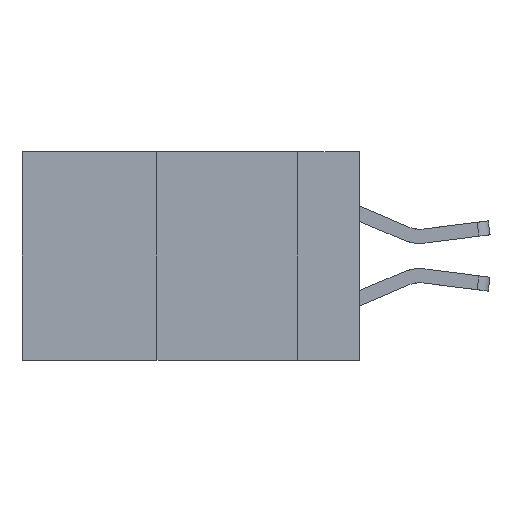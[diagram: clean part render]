
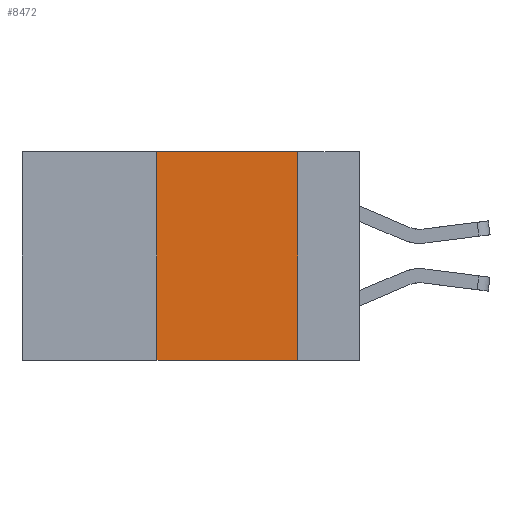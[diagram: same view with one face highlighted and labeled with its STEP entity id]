
A CAD part, left-side view. The second image highlights one B-rep face of the part: STEP entity #8472.
In plain terms, the highlighted planar face has unit normal (-1, 0, 0).
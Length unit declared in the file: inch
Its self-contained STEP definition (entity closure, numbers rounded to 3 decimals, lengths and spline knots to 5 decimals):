
#332 = DIRECTION ( 'NONE',  ( 0., 0., 1. ) ) ;
#389 = DIRECTION ( 'NONE',  ( 0., 0., -1. ) ) ;
#1314 = EDGE_CURVE ( 'NONE', #3086, #7389, #4109, .T. ) ;
#1428 = ORIENTED_EDGE ( 'NONE', *, *, #9769, .F. ) ;
#1453 = VERTEX_POINT ( 'NONE', #2258 ) ;
#2258 = CARTESIAN_POINT ( 'NONE',  ( 0., 0.36, 0. ) ) ;
#2294 = LINE ( 'NONE', #9237, #9039 ) ;
#3086 = VERTEX_POINT ( 'NONE', #4853 ) ;
#3534 = EDGE_CURVE ( 'NONE', #3086, #1453, #8638, .T. ) ;
#3850 = ORIENTED_EDGE ( 'NONE', *, *, #1314, .T. ) ;
#3975 = DIRECTION ( 'NONE',  ( 0., -1., 0. ) ) ;
#4109 = LINE ( 'NONE', #9462, #5399 ) ;
#4118 = CARTESIAN_POINT ( 'NONE',  ( 0., 0.6, 0. ) ) ;
#4625 = DIRECTION ( 'NONE',  ( 0., 0., -1. ) ) ;
#4808 = CARTESIAN_POINT ( 'NONE',  ( 0., 0.11, -0.37 ) ) ;
#4853 = CARTESIAN_POINT ( 'NONE',  ( 0., 0.36, -0.37 ) ) ;
#4981 = LINE ( 'NONE', #5842, #8433 ) ;
#5399 = VECTOR ( 'NONE', #6715, 39.37008 ) ;
#5842 = CARTESIAN_POINT ( 'NONE',  ( 0., 0.6, 0. ) ) ;
#6715 = DIRECTION ( 'NONE',  ( 0., -1., 0. ) ) ;
#6769 = ORIENTED_EDGE ( 'NONE', *, *, #9704, .F. ) ;
#6993 = ORIENTED_EDGE ( 'NONE', *, *, #3534, .F. ) ;
#7389 = VERTEX_POINT ( 'NONE', #4808 ) ;
#8433 = VECTOR ( 'NONE', #3975, 39.37008 ) ;
#8457 = VERTEX_POINT ( 'NONE', #10079 ) ;
#8472 = ADVANCED_FACE ( 'NONE', ( #11332 ), #8593, .F. ) ;
#8576 = CARTESIAN_POINT ( 'NONE',  ( 0., 0.36, 0. ) ) ;
#8593 = PLANE ( 'NONE',  #8844 ) ;
#8638 = LINE ( 'NONE', #8576, #11670 ) ;
#8844 = AXIS2_PLACEMENT_3D ( 'NONE', #4118, #11323, #389 ) ;
#9039 = VECTOR ( 'NONE', #4625, 39.37008 ) ;
#9237 = CARTESIAN_POINT ( 'NONE',  ( 0., 0.11, 0. ) ) ;
#9462 = CARTESIAN_POINT ( 'NONE',  ( 0., 0.6, -0.37 ) ) ;
#9704 = EDGE_CURVE ( 'NONE', #8457, #7389, #2294, .T. ) ;
#9769 = EDGE_CURVE ( 'NONE', #1453, #8457, #4981, .T. ) ;
#10079 = CARTESIAN_POINT ( 'NONE',  ( 0., 0.11, 0. ) ) ;
#11323 = DIRECTION ( 'NONE',  ( 1., 0., 0. ) ) ;
#11332 = FACE_OUTER_BOUND ( 'NONE', #11376, .T. ) ;
#11376 = EDGE_LOOP ( 'NONE', ( #6769, #1428, #6993, #3850 ) ) ;
#11670 = VECTOR ( 'NONE', #332, 39.37008 ) ;
